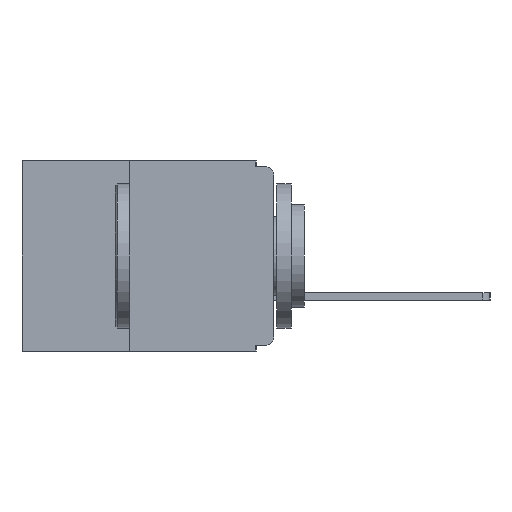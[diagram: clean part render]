
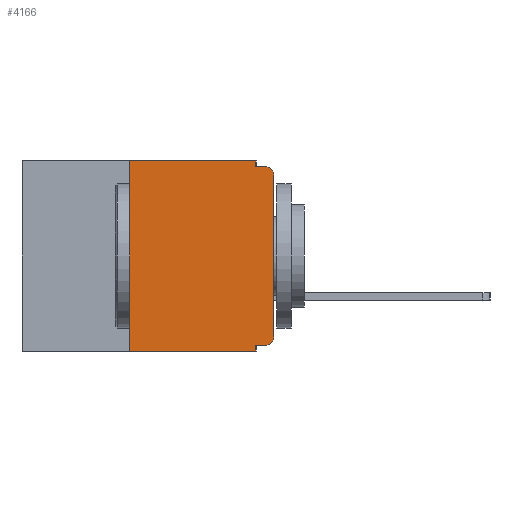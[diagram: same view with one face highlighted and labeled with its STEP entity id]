
A CAD part, left-side view. The second image highlights one B-rep face of the part: STEP entity #4166.
In plain terms, the highlighted planar face has unit normal (-1, 0, 0).
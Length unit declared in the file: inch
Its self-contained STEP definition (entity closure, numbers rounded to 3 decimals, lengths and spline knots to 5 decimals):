
#184 = LINE ( 'NONE', #12569, #12948 ) ;
#850 = EDGE_CURVE ( 'NONE', #20679, #20622, #3877, .T. ) ;
#1003 = CARTESIAN_POINT ( 'NONE',  ( 0., 0., -0.025 ) ) ;
#1466 = LINE ( 'NONE', #6075, #9324 ) ;
#1714 = ORIENTED_EDGE ( 'NONE', *, *, #6054, .F. ) ;
#1902 = ORIENTED_EDGE ( 'NONE', *, *, #6250, .F. ) ;
#1946 = DIRECTION ( 'NONE',  ( 0., -1., 0. ) ) ;
#2420 = DIRECTION ( 'NONE',  ( -1., 0., 0. ) ) ;
#2548 = DIRECTION ( 'NONE',  ( 0., 0., -1. ) ) ;
#2638 = EDGE_CURVE ( 'NONE', #3757, #3603, #17911, .T. ) ;
#2639 = ORIENTED_EDGE ( 'NONE', *, *, #2720, .T. ) ;
#2720 = EDGE_CURVE ( 'NONE', #3663, #20716, #7635, .T. ) ;
#3146 = EDGE_CURVE ( 'NONE', #5216, #20716, #12586, .T. ) ;
#3179 = CARTESIAN_POINT ( 'NONE',  ( 0., 0.031, -0.01 ) ) ;
#3286 = ORIENTED_EDGE ( 'NONE', *, *, #9117, .T. ) ;
#3328 = DIRECTION ( 'NONE',  ( 1., 0., 0. ) ) ;
#3603 = VERTEX_POINT ( 'NONE', #9762 ) ;
#3663 = VERTEX_POINT ( 'NONE', #1003 ) ;
#3757 = VERTEX_POINT ( 'NONE', #8619 ) ;
#3816 = LINE ( 'NONE', #10418, #16493 ) ;
#3877 = LINE ( 'NONE', #18688, #11750 ) ;
#4163 = CARTESIAN_POINT ( 'NONE',  ( 0., 0.015, -0.32 ) ) ;
#4166 = ADVANCED_FACE ( 'NONE', ( #9968 ), #12298, .F. ) ;
#4199 = VECTOR ( 'NONE', #7121, 39.37008 ) ;
#4413 = VECTOR ( 'NONE', #18976, 39.37008 ) ;
#4836 = AXIS2_PLACEMENT_3D ( 'NONE', #12430, #2420, #14040 ) ;
#4865 = CARTESIAN_POINT ( 'NONE',  ( 0., 0.031, -0.33 ) ) ;
#5188 = VERTEX_POINT ( 'NONE', #19510 ) ;
#5216 = VERTEX_POINT ( 'NONE', #3179 ) ;
#6054 = EDGE_CURVE ( 'NONE', #18986, #20679, #3816, .T. ) ;
#6075 = CARTESIAN_POINT ( 'NONE',  ( 0., 0., 0. ) ) ;
#6250 = EDGE_CURVE ( 'NONE', #3603, #5216, #184, .T. ) ;
#7121 = DIRECTION ( 'NONE',  ( 0., -1., 0. ) ) ;
#7409 = CARTESIAN_POINT ( 'NONE',  ( 0., 0., -0.01 ) ) ;
#7635 = CIRCLE ( 'NONE', #20401, 0.015 ) ;
#7770 = DIRECTION ( 'NONE',  ( 0., 0., 1. ) ) ;
#8403 = CARTESIAN_POINT ( 'NONE',  ( 0., 0.031, -0.32 ) ) ;
#8619 = CARTESIAN_POINT ( 'NONE',  ( 0., 0.25, 0. ) ) ;
#9117 = EDGE_CURVE ( 'NONE', #11402, #3663, #1466, .T. ) ;
#9248 = VECTOR ( 'NONE', #1946, 39.37008 ) ;
#9277 = AXIS2_PLACEMENT_3D ( 'NONE', #12035, #3328, #11802 ) ;
#9324 = VECTOR ( 'NONE', #7770, 39.37008 ) ;
#9347 = LINE ( 'NONE', #13038, #13705 ) ;
#9450 = LINE ( 'NONE', #17362, #4413 ) ;
#9762 = CARTESIAN_POINT ( 'NONE',  ( 0., 0.031, 0. ) ) ;
#9968 = FACE_OUTER_BOUND ( 'NONE', #20485, .T. ) ;
#10418 = CARTESIAN_POINT ( 'NONE',  ( 0., 0., -0.32 ) ) ;
#11233 = ORIENTED_EDGE ( 'NONE', *, *, #850, .F. ) ;
#11402 = VERTEX_POINT ( 'NONE', #19988 ) ;
#11750 = VECTOR ( 'NONE', #17910, 39.37008 ) ;
#11802 = DIRECTION ( 'NONE',  ( 0., 0., -1. ) ) ;
#12035 = CARTESIAN_POINT ( 'NONE',  ( 0., 0.437, 0. ) ) ;
#12067 = DIRECTION ( 'NONE',  ( 0., 1., 0. ) ) ;
#12298 = PLANE ( 'NONE',  #9277 ) ;
#12430 = CARTESIAN_POINT ( 'NONE',  ( 0., 0.015, -0.305 ) ) ;
#12569 = CARTESIAN_POINT ( 'NONE',  ( 0., 0.031, 0. ) ) ;
#12586 = LINE ( 'NONE', #7409, #4199 ) ;
#12836 = EDGE_CURVE ( 'NONE', #18986, #11402, #17328, .T. ) ;
#12948 = VECTOR ( 'NONE', #2548, 39.37008 ) ;
#13038 = CARTESIAN_POINT ( 'NONE',  ( 0., 0.437, -0.33 ) ) ;
#13705 = VECTOR ( 'NONE', #21064, 39.37008 ) ;
#14040 = DIRECTION ( 'NONE',  ( 0., 0., -1. ) ) ;
#14577 = EDGE_CURVE ( 'NONE', #5188, #3757, #9450, .T. ) ;
#14706 = ORIENTED_EDGE ( 'NONE', *, *, #20541, .T. ) ;
#15099 = ORIENTED_EDGE ( 'NONE', *, *, #14577, .F. ) ;
#16493 = VECTOR ( 'NONE', #12067, 39.37008 ) ;
#16576 = ORIENTED_EDGE ( 'NONE', *, *, #3146, .F. ) ;
#17328 = CIRCLE ( 'NONE', #4836, 0.015 ) ;
#17362 = CARTESIAN_POINT ( 'NONE',  ( 0., 0.25, -0.33 ) ) ;
#17910 = DIRECTION ( 'NONE',  ( 0., 0., -1. ) ) ;
#17911 = LINE ( 'NONE', #19055, #9248 ) ;
#18149 = DIRECTION ( 'NONE',  ( 0., 0., -1. ) ) ;
#18586 = CARTESIAN_POINT ( 'NONE',  ( 0., 0.015, -0.025 ) ) ;
#18688 = CARTESIAN_POINT ( 'NONE',  ( 0., 0.031, -0.33 ) ) ;
#18976 = DIRECTION ( 'NONE',  ( 0., 0., 1. ) ) ;
#18986 = VERTEX_POINT ( 'NONE', #4163 ) ;
#19055 = CARTESIAN_POINT ( 'NONE',  ( 0., 0.437, 0. ) ) ;
#19214 = DIRECTION ( 'NONE',  ( -1., 0., 0. ) ) ;
#19342 = ORIENTED_EDGE ( 'NONE', *, *, #2638, .F. ) ;
#19510 = CARTESIAN_POINT ( 'NONE',  ( 0., 0.25, -0.33 ) ) ;
#19683 = ORIENTED_EDGE ( 'NONE', *, *, #12836, .T. ) ;
#19864 = CARTESIAN_POINT ( 'NONE',  ( 0., 0.015, -0.01 ) ) ;
#19988 = CARTESIAN_POINT ( 'NONE',  ( 0., 0., -0.305 ) ) ;
#20401 = AXIS2_PLACEMENT_3D ( 'NONE', #18586, #19214, #18149 ) ;
#20485 = EDGE_LOOP ( 'NONE', ( #3286, #2639, #16576, #1902, #19342, #15099, #14706, #11233, #1714, #19683 ) ) ;
#20541 = EDGE_CURVE ( 'NONE', #5188, #20622, #9347, .T. ) ;
#20622 = VERTEX_POINT ( 'NONE', #4865 ) ;
#20679 = VERTEX_POINT ( 'NONE', #8403 ) ;
#20716 = VERTEX_POINT ( 'NONE', #19864 ) ;
#21064 = DIRECTION ( 'NONE',  ( 0., -1., 0. ) ) ;
